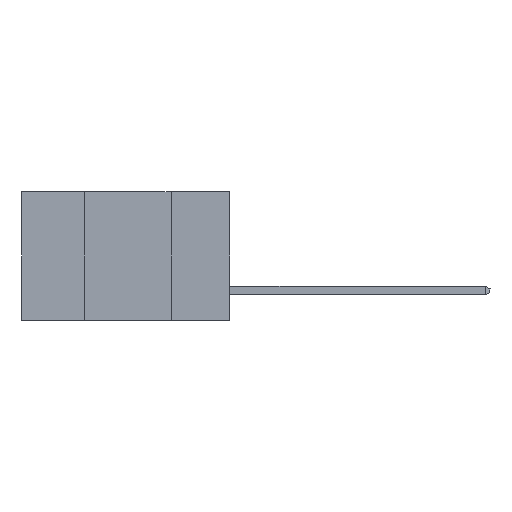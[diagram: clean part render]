
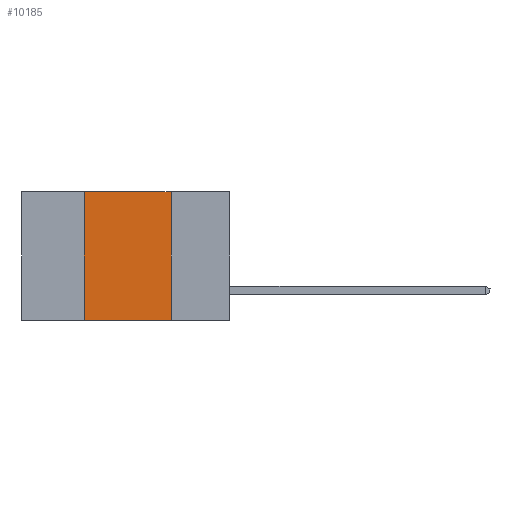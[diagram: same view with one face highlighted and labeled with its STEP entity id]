
A CAD part, left-side view. The second image highlights one B-rep face of the part: STEP entity #10185.
In plain terms, the highlighted planar face has unit normal (-1, 0, 0).
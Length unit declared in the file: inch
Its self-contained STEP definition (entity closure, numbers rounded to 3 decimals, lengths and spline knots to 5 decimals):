
#26 = VECTOR ( 'NONE', #12790, 39.37008 ) ;
#846 = AXIS2_PLACEMENT_3D ( 'NONE', #10898, #3095, #1851 ) ;
#1753 = LINE ( 'NONE', #6347, #13383 ) ;
#1847 = VERTEX_POINT ( 'NONE', #11978 ) ;
#1851 = DIRECTION ( 'NONE',  ( 0., 0., -1. ) ) ;
#2898 = CARTESIAN_POINT ( 'NONE',  ( 0., 0.42, 0. ) ) ;
#3095 = DIRECTION ( 'NONE',  ( 1., 0., 0. ) ) ;
#3312 = FACE_OUTER_BOUND ( 'NONE', #4545, .T. ) ;
#3683 = DIRECTION ( 'NONE',  ( 0., -1., 0. ) ) ;
#4201 = ORIENTED_EDGE ( 'NONE', *, *, #10177, .F. ) ;
#4545 = EDGE_LOOP ( 'NONE', ( #8406, #8993, #4201, #10311 ) ) ;
#4892 = VECTOR ( 'NONE', #12040, 39.37008 ) ;
#4981 = LINE ( 'NONE', #11847, #26 ) ;
#5418 = VECTOR ( 'NONE', #3683, 39.37008 ) ;
#6347 = CARTESIAN_POINT ( 'NONE',  ( 0., 0.6, 0. ) ) ;
#6382 = CARTESIAN_POINT ( 'NONE',  ( 0., 0.42, 0. ) ) ;
#7011 = LINE ( 'NONE', #6382, #4892 ) ;
#7382 = PLANE ( 'NONE',  #846 ) ;
#7471 = DIRECTION ( 'NONE',  ( 0., -1., 0. ) ) ;
#7699 = EDGE_CURVE ( 'NONE', #1847, #8816, #4981, .T. ) ;
#7700 = LINE ( 'NONE', #11616, #5418 ) ;
#8247 = VERTEX_POINT ( 'NONE', #10440 ) ;
#8406 = ORIENTED_EDGE ( 'NONE', *, *, #7699, .F. ) ;
#8816 = VERTEX_POINT ( 'NONE', #13792 ) ;
#8961 = EDGE_CURVE ( 'NONE', #10139, #1847, #1753, .T. ) ;
#8993 = ORIENTED_EDGE ( 'NONE', *, *, #8961, .F. ) ;
#9785 = EDGE_CURVE ( 'NONE', #8247, #8816, #7700, .T. ) ;
#10139 = VERTEX_POINT ( 'NONE', #2898 ) ;
#10177 = EDGE_CURVE ( 'NONE', #8247, #10139, #7011, .T. ) ;
#10185 = ADVANCED_FACE ( 'NONE', ( #3312 ), #7382, .F. ) ;
#10311 = ORIENTED_EDGE ( 'NONE', *, *, #9785, .T. ) ;
#10440 = CARTESIAN_POINT ( 'NONE',  ( 0., 0.42, -0.37 ) ) ;
#10898 = CARTESIAN_POINT ( 'NONE',  ( 0., 0.6, 0. ) ) ;
#11616 = CARTESIAN_POINT ( 'NONE',  ( 0., 0.6, -0.37 ) ) ;
#11847 = CARTESIAN_POINT ( 'NONE',  ( 0., 0.17, 0. ) ) ;
#11978 = CARTESIAN_POINT ( 'NONE',  ( 0., 0.17, 0. ) ) ;
#12040 = DIRECTION ( 'NONE',  ( 0., 0., 1. ) ) ;
#12790 = DIRECTION ( 'NONE',  ( 0., 0., -1. ) ) ;
#13383 = VECTOR ( 'NONE', #7471, 39.37008 ) ;
#13792 = CARTESIAN_POINT ( 'NONE',  ( 0., 0.17, -0.37 ) ) ;
